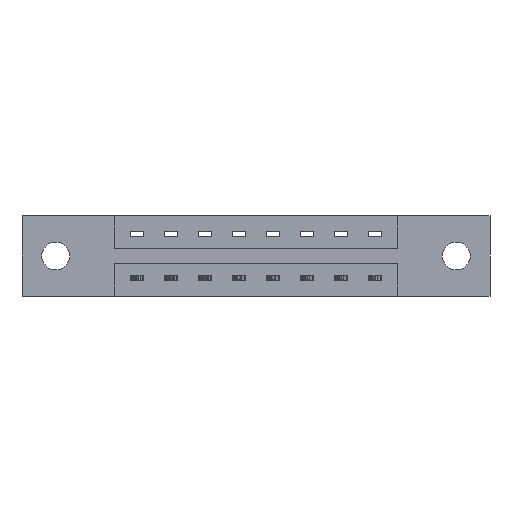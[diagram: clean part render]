
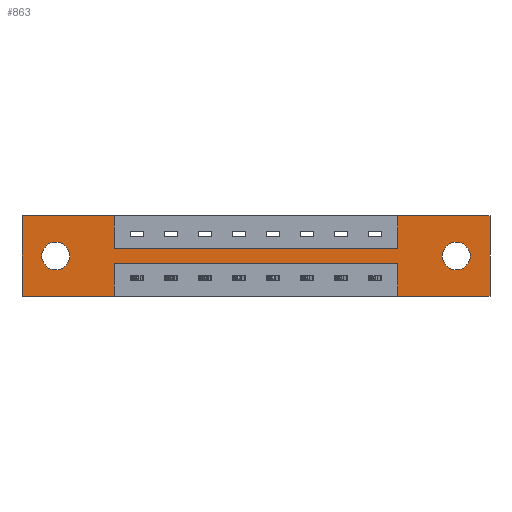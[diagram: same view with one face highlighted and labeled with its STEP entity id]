
A CAD part, front view. The second image highlights one B-rep face of the part: STEP entity #863.
In plain terms, the highlighted planar face has unit normal (0, -1, 0).
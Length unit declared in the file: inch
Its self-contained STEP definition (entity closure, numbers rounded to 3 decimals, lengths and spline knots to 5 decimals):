
#6 = VERTEX_POINT ( 'NONE', #859 ) ;
#7 = VECTOR ( 'NONE', #2095, 39.37008 ) ;
#84 = DIRECTION ( 'NONE',  ( 0., 1., 0. ) ) ;
#92 = LINE ( 'NONE', #9369, #733 ) ;
#107 = CARTESIAN_POINT ( 'NONE',  ( 0., 0., 0. ) ) ;
#169 = VERTEX_POINT ( 'NONE', #9127 ) ;
#171 = EDGE_CURVE ( 'NONE', #5143, #3907, #1655, .T. ) ;
#250 = CARTESIAN_POINT ( 'NONE',  ( 0.425, 0., -0.15 ) ) ;
#274 = EDGE_CURVE ( 'NONE', #2829, #5143, #4897, .T. ) ;
#303 = DIRECTION ( 'NONE',  ( 0., 0., -1. ) ) ;
#608 = CARTESIAN_POINT ( 'NONE',  ( 0.425, 0., -0.22 ) ) ;
#635 = CARTESIAN_POINT ( 'NONE',  ( 0.425, 0., 0. ) ) ;
#733 = VECTOR ( 'NONE', #6882, 39.37008 ) ;
#789 = EDGE_LOOP ( 'NONE', ( #6008, #6049, #1910, #5800, #814, #2526, #4546, #8657, #9509, #1575, #8207, #3874 ) ) ;
#794 = VERTEX_POINT ( 'NONE', #6495 ) ;
#814 = ORIENTED_EDGE ( 'NONE', *, *, #8105, .F. ) ;
#820 = CARTESIAN_POINT ( 'NONE',  ( 0., 0., 0. ) ) ;
#859 = CARTESIAN_POINT ( 'NONE',  ( 0., 0., -0.37 ) ) ;
#863 = ADVANCED_FACE ( 'NONE', ( #2410, #8247, #3645 ), #7484, .T. ) ;
#902 = CARTESIAN_POINT ( 'NONE',  ( 0., 0., -0.37 ) ) ;
#939 = VERTEX_POINT ( 'NONE', #5096 ) ;
#1042 = EDGE_CURVE ( 'NONE', #3907, #10262, #4877, .T. ) ;
#1209 = EDGE_CURVE ( 'NONE', #3304, #6, #6484, .T. ) ;
#1292 = EDGE_LOOP ( 'NONE', ( #6302, #9967 ) ) ;
#1359 = VECTOR ( 'NONE', #4985, 39.37008 ) ;
#1392 = VECTOR ( 'NONE', #3369, 39.37008 ) ;
#1575 = ORIENTED_EDGE ( 'NONE', *, *, #1748, .F. ) ;
#1655 = LINE ( 'NONE', #250, #7352 ) ;
#1748 = EDGE_CURVE ( 'NONE', #9911, #2829, #3999, .T. ) ;
#1910 = ORIENTED_EDGE ( 'NONE', *, *, #9380, .F. ) ;
#2005 = EDGE_CURVE ( 'NONE', #9243, #169, #7831, .T. ) ;
#2009 = EDGE_CURVE ( 'NONE', #794, #8814, #7692, .T. ) ;
#2095 = DIRECTION ( 'NONE',  ( 0., 0., -1. ) ) ;
#2214 = VECTOR ( 'NONE', #10053, 39.37008 ) ;
#2275 = ORIENTED_EDGE ( 'NONE', *, *, #7462, .T. ) ;
#2312 = DIRECTION ( 'NONE',  ( 0., 0., -1. ) ) ;
#2346 = LINE ( 'NONE', #9415, #2214 ) ;
#2383 = AXIS2_PLACEMENT_3D ( 'NONE', #2684, #9084, #9756 ) ;
#2410 = FACE_BOUND ( 'NONE', #8026, .T. ) ;
#2416 = LINE ( 'NONE', #107, #1392 ) ;
#2526 = ORIENTED_EDGE ( 'NONE', *, *, #8502, .F. ) ;
#2646 = CARTESIAN_POINT ( 'NONE',  ( 1.999, 0., -0.185 ) ) ;
#2684 = CARTESIAN_POINT ( 'NONE',  ( 0.155, 0., -0.185 ) ) ;
#2829 = VERTEX_POINT ( 'NONE', #635 ) ;
#2858 = DIRECTION ( 'NONE',  ( 0., 0., -1. ) ) ;
#2865 = CIRCLE ( 'NONE', #7422, 0.064 ) ;
#2868 = EDGE_CURVE ( 'NONE', #9993, #8024, #3726, .T. ) ;
#3150 = DIRECTION ( 'NONE',  ( 0., 0., 1. ) ) ;
#3179 = CARTESIAN_POINT ( 'NONE',  ( 1.729, 0., 0. ) ) ;
#3268 = DIRECTION ( 'NONE',  ( 1., 0., 0. ) ) ;
#3304 = VERTEX_POINT ( 'NONE', #5968 ) ;
#3369 = DIRECTION ( 'NONE',  ( 0., 0., 1. ) ) ;
#3539 = CARTESIAN_POINT ( 'NONE',  ( 0., 0., 0. ) ) ;
#3620 = CARTESIAN_POINT ( 'NONE',  ( 1.729, 0., 0. ) ) ;
#3645 = FACE_OUTER_BOUND ( 'NONE', #789, .T. ) ;
#3726 = CIRCLE ( 'NONE', #4647, 0.064 ) ;
#3752 = CARTESIAN_POINT ( 'NONE',  ( 0.425, 0., 0. ) ) ;
#3788 = AXIS2_PLACEMENT_3D ( 'NONE', #9630, #84, #6479 ) ;
#3855 = DIRECTION ( 'NONE',  ( 0., 1., 0. ) ) ;
#3874 = ORIENTED_EDGE ( 'NONE', *, *, #1209, .F. ) ;
#3907 = VERTEX_POINT ( 'NONE', #6292 ) ;
#3999 = LINE ( 'NONE', #820, #6213 ) ;
#4034 = AXIS2_PLACEMENT_3D ( 'NONE', #9907, #7586, #303 ) ;
#4476 = CARTESIAN_POINT ( 'NONE',  ( 1.999, 0., -0.121 ) ) ;
#4546 = ORIENTED_EDGE ( 'NONE', *, *, #1042, .F. ) ;
#4647 = AXIS2_PLACEMENT_3D ( 'NONE', #10172, #3855, #2312 ) ;
#4798 = LINE ( 'NONE', #5922, #7 ) ;
#4863 = EDGE_CURVE ( 'NONE', #6, #9911, #2416, .T. ) ;
#4877 = LINE ( 'NONE', #3179, #9731 ) ;
#4897 = LINE ( 'NONE', #3752, #8883 ) ;
#4985 = DIRECTION ( 'NONE',  ( -1., 0., 0. ) ) ;
#5037 = CARTESIAN_POINT ( 'NONE',  ( 0.155, 0., -0.249 ) ) ;
#5096 = CARTESIAN_POINT ( 'NONE',  ( 2.154, 0., 0. ) ) ;
#5143 = VERTEX_POINT ( 'NONE', #7046 ) ;
#5347 = DIRECTION ( 'NONE',  ( 0., 0., 1. ) ) ;
#5387 = CARTESIAN_POINT ( 'NONE',  ( 1.729, 0., -0.37 ) ) ;
#5488 = VECTOR ( 'NONE', #7173, 39.37008 ) ;
#5618 = CARTESIAN_POINT ( 'NONE',  ( 2.154, 0., -0.37 ) ) ;
#5645 = EDGE_CURVE ( 'NONE', #9977, #8812, #92, .T. ) ;
#5800 = ORIENTED_EDGE ( 'NONE', *, *, #5645, .F. ) ;
#5922 = CARTESIAN_POINT ( 'NONE',  ( 0.425, 0., -0.37 ) ) ;
#5936 = EDGE_CURVE ( 'NONE', #169, #9243, #6350, .T. ) ;
#5968 = CARTESIAN_POINT ( 'NONE',  ( 0.425, 0., -0.37 ) ) ;
#6008 = ORIENTED_EDGE ( 'NONE', *, *, #10070, .F. ) ;
#6049 = ORIENTED_EDGE ( 'NONE', *, *, #2009, .F. ) ;
#6153 = CARTESIAN_POINT ( 'NONE',  ( 1.999, 0., -0.249 ) ) ;
#6213 = VECTOR ( 'NONE', #3268, 39.37008 ) ;
#6292 = CARTESIAN_POINT ( 'NONE',  ( 1.729, 0., -0.15 ) ) ;
#6302 = ORIENTED_EDGE ( 'NONE', *, *, #5936, .T. ) ;
#6350 = CIRCLE ( 'NONE', #3788, 0.064 ) ;
#6479 = DIRECTION ( 'NONE',  ( 0., 0., 1. ) ) ;
#6484 = LINE ( 'NONE', #902, #5488 ) ;
#6495 = CARTESIAN_POINT ( 'NONE',  ( 1.729, 0., -0.22 ) ) ;
#6689 = DIRECTION ( 'NONE',  ( 0., 0., -1. ) ) ;
#6831 = CARTESIAN_POINT ( 'NONE',  ( 1.729, 0., -0.37 ) ) ;
#6882 = DIRECTION ( 'NONE',  ( -1., 0., 0. ) ) ;
#7046 = CARTESIAN_POINT ( 'NONE',  ( 0.425, 0., -0.15 ) ) ;
#7173 = DIRECTION ( 'NONE',  ( -1., 0., 0. ) ) ;
#7352 = VECTOR ( 'NONE', #8363, 39.37008 ) ;
#7415 = VECTOR ( 'NONE', #8574, 39.37008 ) ;
#7422 = AXIS2_PLACEMENT_3D ( 'NONE', #2646, #9816, #6689 ) ;
#7462 = EDGE_CURVE ( 'NONE', #8024, #9993, #2865, .T. ) ;
#7484 = PLANE ( 'NONE',  #4034 ) ;
#7586 = DIRECTION ( 'NONE',  ( 0., -1., 0. ) ) ;
#7692 = LINE ( 'NONE', #8960, #1359 ) ;
#7831 = CIRCLE ( 'NONE', #2383, 0.064 ) ;
#8024 = VERTEX_POINT ( 'NONE', #6153 ) ;
#8026 = EDGE_LOOP ( 'NONE', ( #9158, #2275 ) ) ;
#8105 = EDGE_CURVE ( 'NONE', #939, #9977, #8551, .T. ) ;
#8207 = ORIENTED_EDGE ( 'NONE', *, *, #4863, .F. ) ;
#8247 = FACE_BOUND ( 'NONE', #1292, .T. ) ;
#8363 = DIRECTION ( 'NONE',  ( 1., 0., 0. ) ) ;
#8502 = EDGE_CURVE ( 'NONE', #10262, #939, #2346, .T. ) ;
#8551 = LINE ( 'NONE', #10018, #7415 ) ;
#8574 = DIRECTION ( 'NONE',  ( 0., 0., -1. ) ) ;
#8657 = ORIENTED_EDGE ( 'NONE', *, *, #171, .F. ) ;
#8812 = VERTEX_POINT ( 'NONE', #5387 ) ;
#8814 = VERTEX_POINT ( 'NONE', #608 ) ;
#8883 = VECTOR ( 'NONE', #2858, 39.37008 ) ;
#8960 = CARTESIAN_POINT ( 'NONE',  ( 0.425, 0., -0.22 ) ) ;
#9084 = DIRECTION ( 'NONE',  ( 0., 1., 0. ) ) ;
#9127 = CARTESIAN_POINT ( 'NONE',  ( 0.155, 0., -0.121 ) ) ;
#9158 = ORIENTED_EDGE ( 'NONE', *, *, #2868, .T. ) ;
#9243 = VERTEX_POINT ( 'NONE', #5037 ) ;
#9293 = VECTOR ( 'NONE', #5347, 39.37008 ) ;
#9369 = CARTESIAN_POINT ( 'NONE',  ( 0., 0., -0.37 ) ) ;
#9380 = EDGE_CURVE ( 'NONE', #8812, #794, #9542, .T. ) ;
#9415 = CARTESIAN_POINT ( 'NONE',  ( 0., 0., 0. ) ) ;
#9509 = ORIENTED_EDGE ( 'NONE', *, *, #274, .F. ) ;
#9542 = LINE ( 'NONE', #6831, #9293 ) ;
#9630 = CARTESIAN_POINT ( 'NONE',  ( 0.155, 0., -0.185 ) ) ;
#9731 = VECTOR ( 'NONE', #3150, 39.37008 ) ;
#9756 = DIRECTION ( 'NONE',  ( 0., 0., 1. ) ) ;
#9816 = DIRECTION ( 'NONE',  ( 0., 1., 0. ) ) ;
#9907 = CARTESIAN_POINT ( 'NONE',  ( 0., 0., -0.37 ) ) ;
#9911 = VERTEX_POINT ( 'NONE', #3539 ) ;
#9967 = ORIENTED_EDGE ( 'NONE', *, *, #2005, .T. ) ;
#9977 = VERTEX_POINT ( 'NONE', #5618 ) ;
#9993 = VERTEX_POINT ( 'NONE', #4476 ) ;
#10018 = CARTESIAN_POINT ( 'NONE',  ( 2.154, 0., 0. ) ) ;
#10053 = DIRECTION ( 'NONE',  ( 1., 0., 0. ) ) ;
#10070 = EDGE_CURVE ( 'NONE', #8814, #3304, #4798, .T. ) ;
#10172 = CARTESIAN_POINT ( 'NONE',  ( 1.999, 0., -0.185 ) ) ;
#10262 = VERTEX_POINT ( 'NONE', #3620 ) ;
